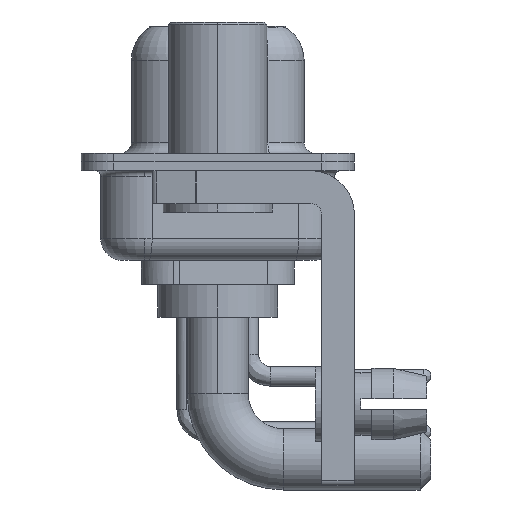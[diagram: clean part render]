
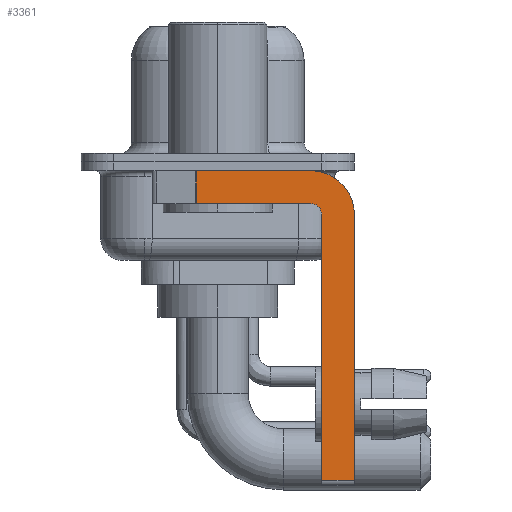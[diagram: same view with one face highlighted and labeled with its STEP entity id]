
A CAD part, left-side view. The second image highlights one B-rep face of the part: STEP entity #3361.
In plain terms, the highlighted planar face has unit normal (-1, 0, 0).
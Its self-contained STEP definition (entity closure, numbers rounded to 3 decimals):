
#171 = ORIENTED_EDGE ( 'NONE', *, *, #2268, .F. ) ;
#588 = ORIENTED_EDGE ( 'NONE', *, *, #16443, .F. ) ;
#897 = ORIENTED_EDGE ( 'NONE', *, *, #5886, .F. ) ;
#1613 = PLANE ( 'NONE',  #18615 ) ;
#1880 = CARTESIAN_POINT ( 'NONE',  ( -2.9, -6.25, -14.55 ) ) ;
#2268 = EDGE_CURVE ( 'NONE', #17073, #20446, #8170, .T. ) ;
#2489 = EDGE_CURVE ( 'NONE', #14301, #21184, #4035, .T. ) ;
#2492 = CARTESIAN_POINT ( 'NONE',  ( -2.9, 0.978, -0.4 ) ) ;
#3281 = DIRECTION ( 'NONE',  ( 0., 1., 0. ) ) ;
#3314 = VERTEX_POINT ( 'NONE', #2492 ) ;
#3361 = ADVANCED_FACE ( 'NONE', ( #4436 ), #1613, .F. ) ;
#4035 = LINE ( 'NONE', #18745, #17595 ) ;
#4436 = FACE_OUTER_BOUND ( 'NONE', #12395, .T. ) ;
#4545 = DIRECTION ( 'NONE',  ( 0., 0., -1. ) ) ;
#4607 = DIRECTION ( 'NONE',  ( 0., 0., 1. ) ) ;
#4750 = CARTESIAN_POINT ( 'NONE',  ( -2.9, -6.25, -2.4 ) ) ;
#5084 = DIRECTION ( 'NONE',  ( 0., -1., 0. ) ) ;
#5299 = LINE ( 'NONE', #16672, #15342 ) ;
#5886 = EDGE_CURVE ( 'NONE', #10517, #16553, #16962, .T. ) ;
#6162 = DIRECTION ( 'NONE',  ( 0., 0., -1. ) ) ;
#6167 = DIRECTION ( 'NONE',  ( 0., 0., 1. ) ) ;
#6235 = DIRECTION ( 'NONE',  ( -1., 0., 0. ) ) ;
#6952 = AXIS2_PLACEMENT_3D ( 'NONE', #18287, #20012, #11487 ) ;
#7394 = LINE ( 'NONE', #12156, #14241 ) ;
#7400 = VECTOR ( 'NONE', #6162, 1000. ) ;
#7501 = CARTESIAN_POINT ( 'NONE',  ( -2.9, -4.75, -14.55 ) ) ;
#7654 = EDGE_CURVE ( 'NONE', #14301, #17191, #14179, .T. ) ;
#8170 = LINE ( 'NONE', #19739, #19669 ) ;
#8227 = DIRECTION ( 'NONE',  ( 1., 0., 0. ) ) ;
#10466 = ORIENTED_EDGE ( 'NONE', *, *, #2489, .F. ) ;
#10517 = VERTEX_POINT ( 'NONE', #18017 ) ;
#10974 = ORIENTED_EDGE ( 'NONE', *, *, #7654, .T. ) ;
#11487 = DIRECTION ( 'NONE',  ( 0., 0., -1. ) ) ;
#11778 = AXIS2_PLACEMENT_3D ( 'NONE', #21053, #6235, #4607 ) ;
#12026 = EDGE_CURVE ( 'NONE', #21184, #17073, #19736, .T. ) ;
#12156 = CARTESIAN_POINT ( 'NONE',  ( -2.9, 0.978, -1.9 ) ) ;
#12395 = EDGE_LOOP ( 'NONE', ( #588, #20307, #171, #21102, #10466, #10974, #13438, #897 ) ) ;
#12559 = CARTESIAN_POINT ( 'NONE',  ( -2.9, -4.25, -14.55 ) ) ;
#13019 = CARTESIAN_POINT ( 'NONE',  ( -2.9, 0.978, -1.9 ) ) ;
#13438 = ORIENTED_EDGE ( 'NONE', *, *, #16595, .F. ) ;
#14159 = EDGE_CURVE ( 'NONE', #3314, #20446, #7394, .T. ) ;
#14179 = LINE ( 'NONE', #12559, #15642 ) ;
#14241 = VECTOR ( 'NONE', #18743, 1000. ) ;
#14301 = VERTEX_POINT ( 'NONE', #7501 ) ;
#15342 = VECTOR ( 'NONE', #5084, 1000. ) ;
#15642 = VECTOR ( 'NONE', #19150, 1000. ) ;
#15698 = CARTESIAN_POINT ( 'NONE',  ( -2.9, -6.25, -2.4 ) ) ;
#16126 = CARTESIAN_POINT ( 'NONE',  ( -2.9, -4.25, -2.4 ) ) ;
#16443 = EDGE_CURVE ( 'NONE', #3314, #10517, #5299, .T. ) ;
#16553 = VERTEX_POINT ( 'NONE', #15698 ) ;
#16595 = EDGE_CURVE ( 'NONE', #16553, #17191, #19681, .T. ) ;
#16672 = CARTESIAN_POINT ( 'NONE',  ( -2.9, 3., -0.4 ) ) ;
#16962 = CIRCLE ( 'NONE', #6952, 2. ) ;
#17073 = VERTEX_POINT ( 'NONE', #19652 ) ;
#17191 = VERTEX_POINT ( 'NONE', #1880 ) ;
#17595 = VECTOR ( 'NONE', #6167, 1000. ) ;
#17597 = CARTESIAN_POINT ( 'NONE',  ( -2.9, -4.75, -2.4 ) ) ;
#18017 = CARTESIAN_POINT ( 'NONE',  ( -2.9, -4.25, -0.4 ) ) ;
#18287 = CARTESIAN_POINT ( 'NONE',  ( -2.9, -4.25, -2.4 ) ) ;
#18615 = AXIS2_PLACEMENT_3D ( 'NONE', #16126, #8227, #4545 ) ;
#18743 = DIRECTION ( 'NONE',  ( 0., 0., -1. ) ) ;
#18745 = CARTESIAN_POINT ( 'NONE',  ( -2.9, -4.75, -14.8 ) ) ;
#19150 = DIRECTION ( 'NONE',  ( 0., -1., 0. ) ) ;
#19652 = CARTESIAN_POINT ( 'NONE',  ( -2.9, -4.25, -1.9 ) ) ;
#19669 = VECTOR ( 'NONE', #3281, 1000. ) ;
#19681 = LINE ( 'NONE', #4750, #7400 ) ;
#19736 = CIRCLE ( 'NONE', #11778, 0.5 ) ;
#19739 = CARTESIAN_POINT ( 'NONE',  ( -2.9, -4.25, -1.9 ) ) ;
#20012 = DIRECTION ( 'NONE',  ( 1., 0., 0. ) ) ;
#20307 = ORIENTED_EDGE ( 'NONE', *, *, #14159, .T. ) ;
#20446 = VERTEX_POINT ( 'NONE', #13019 ) ;
#21053 = CARTESIAN_POINT ( 'NONE',  ( -2.9, -4.25, -2.4 ) ) ;
#21102 = ORIENTED_EDGE ( 'NONE', *, *, #12026, .F. ) ;
#21184 = VERTEX_POINT ( 'NONE', #17597 ) ;
